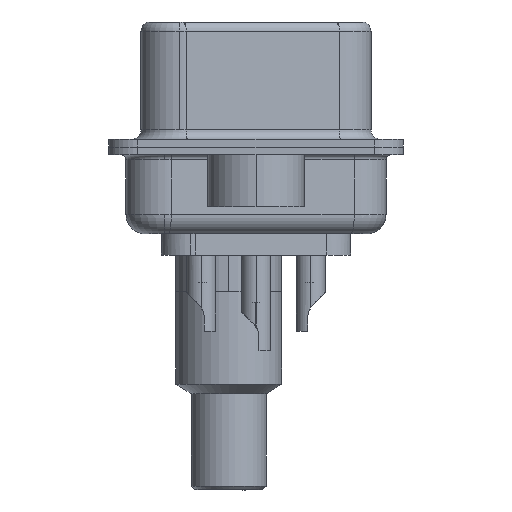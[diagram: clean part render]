
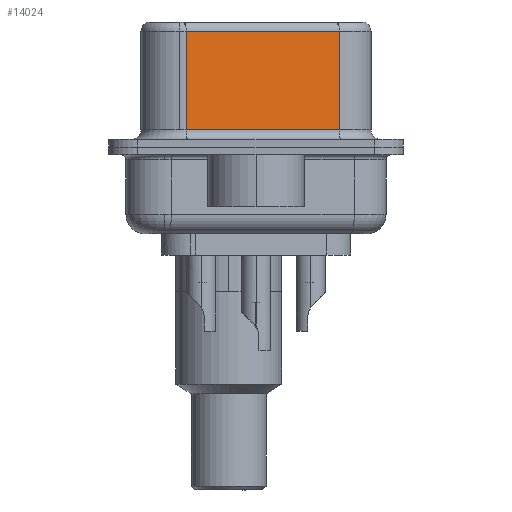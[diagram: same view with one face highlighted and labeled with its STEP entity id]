
A CAD part, left-side view. The second image highlights one B-rep face of the part: STEP entity #14024.
In plain terms, the highlighted planar face has unit normal (-0.985, -0.174, 0).
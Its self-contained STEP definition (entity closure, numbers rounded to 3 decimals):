
#535 = ORIENTED_EDGE ( 'NONE', *, *, #9338, .T. ) ;
#900 = DIRECTION ( 'NONE',  ( 0.174, -0.985, 0. ) ) ;
#1011 = DIRECTION ( 'NONE',  ( 0., 0., -1. ) ) ;
#1130 = VERTEX_POINT ( 'NONE', #29248 ) ;
#2419 = DIRECTION ( 'NONE',  ( -0.174, 0.985, 0. ) ) ;
#2947 = LINE ( 'NONE', #17083, #15226 ) ;
#3097 = LINE ( 'NONE', #3379, #21103 ) ;
#3379 = CARTESIAN_POINT ( 'NONE',  ( 5.132, -4.322, 0.9 ) ) ;
#4329 = ORIENTED_EDGE ( 'NONE', *, *, #14957, .F. ) ;
#4494 = LINE ( 'NONE', #14452, #16773 ) ;
#4728 = ORIENTED_EDGE ( 'NONE', *, *, #11826, .T. ) ;
#4749 = DIRECTION ( 'NONE',  ( -0.174, 0.985, 0. ) ) ;
#7086 = VERTEX_POINT ( 'NONE', #14103 ) ;
#7096 = DIRECTION ( 'NONE',  ( 0., 0., -1. ) ) ;
#8223 = AXIS2_PLACEMENT_3D ( 'NONE', #29315, #17105, #2419 ) ;
#8357 = CARTESIAN_POINT ( 'NONE',  ( 3.73, 3.628, 6.52 ) ) ;
#8974 = EDGE_LOOP ( 'NONE', ( #4329, #535, #4728, #29225 ) ) ;
#9338 = EDGE_CURVE ( 'NONE', #1130, #7086, #2947, .T. ) ;
#11826 = EDGE_CURVE ( 'NONE', #7086, #15799, #30389, .T. ) ;
#12223 = FACE_OUTER_BOUND ( 'NONE', #8974, .T. ) ;
#14024 = ADVANCED_FACE ( 'NONE', ( #12223 ), #31758, .F. ) ;
#14103 = CARTESIAN_POINT ( 'NONE',  ( 3.73, 3.628, 6.02 ) ) ;
#14452 = CARTESIAN_POINT ( 'NONE',  ( 5.132, -4.322, 6.52 ) ) ;
#14957 = EDGE_CURVE ( 'NONE', #1130, #19798, #4494, .T. ) ;
#15226 = VECTOR ( 'NONE', #4749, 1000. ) ;
#15799 = VERTEX_POINT ( 'NONE', #22759 ) ;
#16773 = VECTOR ( 'NONE', #7096, 1000. ) ;
#17083 = CARTESIAN_POINT ( 'NONE',  ( 5.132, -4.322, 6.02 ) ) ;
#17105 = DIRECTION ( 'NONE',  ( 0.985, 0.174, 0. ) ) ;
#17764 = CARTESIAN_POINT ( 'NONE',  ( 5.132, -4.322, 0.9 ) ) ;
#19798 = VERTEX_POINT ( 'NONE', #17764 ) ;
#19893 = EDGE_CURVE ( 'NONE', #15799, #19798, #3097, .T. ) ;
#21103 = VECTOR ( 'NONE', #900, 1000. ) ;
#22759 = CARTESIAN_POINT ( 'NONE',  ( 3.73, 3.628, 0.9 ) ) ;
#23897 = VECTOR ( 'NONE', #1011, 1000. ) ;
#29225 = ORIENTED_EDGE ( 'NONE', *, *, #19893, .T. ) ;
#29248 = CARTESIAN_POINT ( 'NONE',  ( 5.132, -4.322, 6.02 ) ) ;
#29315 = CARTESIAN_POINT ( 'NONE',  ( 5.132, -4.322, 6.52 ) ) ;
#30389 = LINE ( 'NONE', #8357, #23897 ) ;
#31758 = PLANE ( 'NONE',  #8223 ) ;
